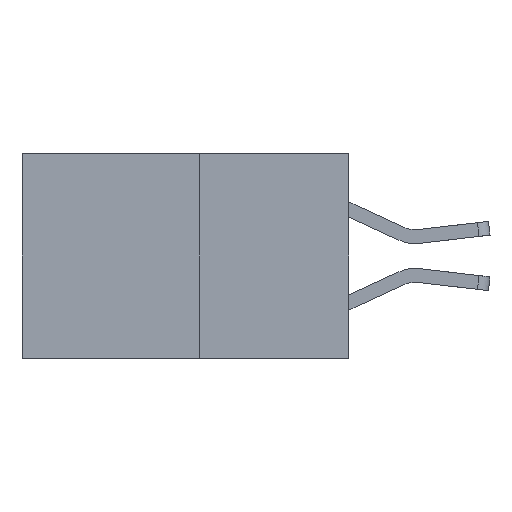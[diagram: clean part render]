
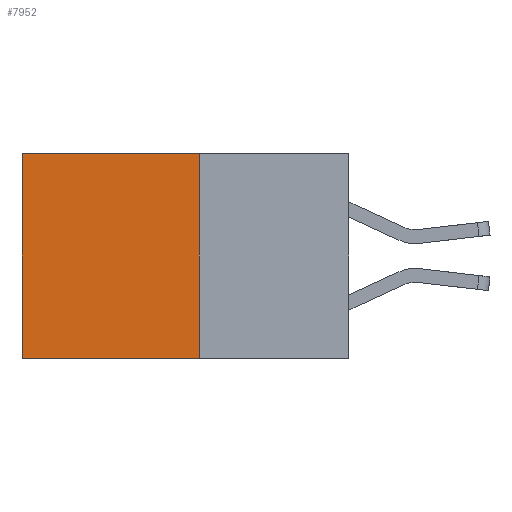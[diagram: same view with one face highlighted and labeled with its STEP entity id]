
A CAD part, left-side view. The second image highlights one B-rep face of the part: STEP entity #7952.
In plain terms, the highlighted planar face has unit normal (-1, 0, 0).
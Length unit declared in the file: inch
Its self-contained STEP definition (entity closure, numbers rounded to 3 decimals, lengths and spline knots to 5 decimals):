
#158 = ORIENTED_EDGE ( 'NONE', *, *, #4315, .T. ) ;
#287 = ORIENTED_EDGE ( 'NONE', *, *, #2667, .F. ) ;
#308 = ORIENTED_EDGE ( 'NONE', *, *, #5402, .F. ) ;
#382 = ORIENTED_EDGE ( 'NONE', *, *, #399, .T. ) ;
#399 = EDGE_CURVE ( 'NONE', #2312, #3951, #6464, .T. ) ;
#671 = CARTESIAN_POINT ( 'NONE',  ( 0.277, 0.27, -0.37 ) ) ;
#1272 = LINE ( 'NONE', #3065, #4748 ) ;
#1555 = FACE_OUTER_BOUND ( 'NONE', #1699, .T. ) ;
#1699 = EDGE_LOOP ( 'NONE', ( #158, #287, #308, #382 ) ) ;
#1798 = DIRECTION ( 'NONE',  ( 0., 0., -1. ) ) ;
#1916 = VECTOR ( 'NONE', #3594, 39.37008 ) ;
#2006 = VERTEX_POINT ( 'NONE', #671 ) ;
#2312 = VERTEX_POINT ( 'NONE', #5914 ) ;
#2667 = EDGE_CURVE ( 'NONE', #2006, #2811, #1272, .T. ) ;
#2811 = VERTEX_POINT ( 'NONE', #3753 ) ;
#3065 = CARTESIAN_POINT ( 'NONE',  ( 0.277, 0.27, -0.37 ) ) ;
#3594 = DIRECTION ( 'NONE',  ( 0., 0., -1. ) ) ;
#3637 = LINE ( 'NONE', #8457, #5379 ) ;
#3753 = CARTESIAN_POINT ( 'NONE',  ( 0.277, 0.59, -0.37 ) ) ;
#3822 = AXIS2_PLACEMENT_3D ( 'NONE', #6368, #6275, #6263 ) ;
#3951 = VERTEX_POINT ( 'NONE', #8382 ) ;
#4039 = CARTESIAN_POINT ( 'NONE',  ( 0.277, 0.27, 0. ) ) ;
#4224 = CARTESIAN_POINT ( 'NONE',  ( 0.277, 0.59, -0.37 ) ) ;
#4315 = EDGE_CURVE ( 'NONE', #3951, #2811, #7378, .T. ) ;
#4748 = VECTOR ( 'NONE', #5015, 39.37008 ) ;
#5015 = DIRECTION ( 'NONE',  ( 0., 1., 0. ) ) ;
#5379 = VECTOR ( 'NONE', #1798, 39.37008 ) ;
#5402 = EDGE_CURVE ( 'NONE', #2312, #2006, #3637, .T. ) ;
#5914 = CARTESIAN_POINT ( 'NONE',  ( 0.277, 0.27, 0. ) ) ;
#6263 = DIRECTION ( 'NONE',  ( 0., 0., -1. ) ) ;
#6275 = DIRECTION ( 'NONE',  ( 1., 0., 0. ) ) ;
#6286 = PLANE ( 'NONE',  #3822 ) ;
#6368 = CARTESIAN_POINT ( 'NONE',  ( 0.277, 0.27, -0.37 ) ) ;
#6464 = LINE ( 'NONE', #4039, #7924 ) ;
#7378 = LINE ( 'NONE', #4224, #1916 ) ;
#7421 = DIRECTION ( 'NONE',  ( 0., 1., 0. ) ) ;
#7924 = VECTOR ( 'NONE', #7421, 39.37008 ) ;
#7952 = ADVANCED_FACE ( 'NONE', ( #1555 ), #6286, .F. ) ;
#8382 = CARTESIAN_POINT ( 'NONE',  ( 0.277, 0.59, 0. ) ) ;
#8457 = CARTESIAN_POINT ( 'NONE',  ( 0.277, 0.27, -0.37 ) ) ;
